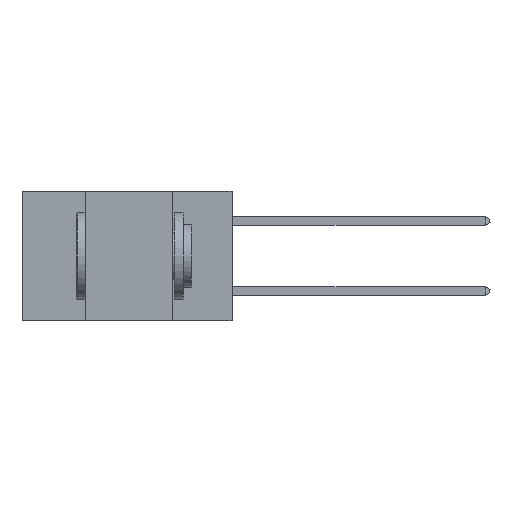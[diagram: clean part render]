
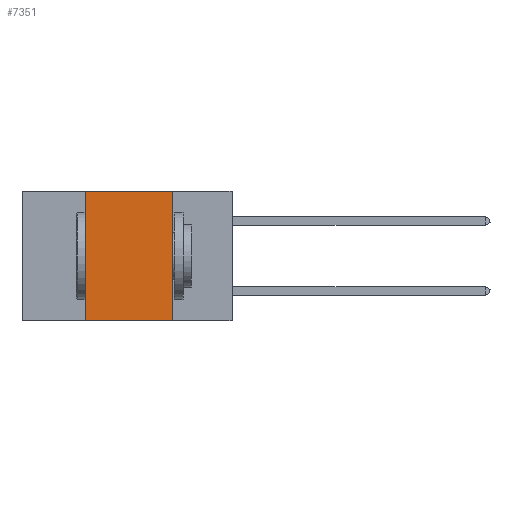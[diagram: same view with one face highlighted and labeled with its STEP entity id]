
A CAD part, left-side view. The second image highlights one B-rep face of the part: STEP entity #7351.
In plain terms, the highlighted planar face has unit normal (-1, 0, 0).
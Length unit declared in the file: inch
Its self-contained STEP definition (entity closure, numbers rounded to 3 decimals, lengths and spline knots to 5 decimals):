
#14 = CARTESIAN_POINT ( 'NONE',  ( 0., 0.6, -0.37 ) ) ;
#1125 = ORIENTED_EDGE ( 'NONE', *, *, #24568, .F. ) ;
#1738 = EDGE_CURVE ( 'NONE', #3433, #2591, #24020, .T. ) ;
#2591 = VERTEX_POINT ( 'NONE', #39258 ) ;
#2994 = VECTOR ( 'NONE', #36422, 39.37008 ) ;
#3433 = VERTEX_POINT ( 'NONE', #27072 ) ;
#7351 = ADVANCED_FACE ( 'NONE', ( #25152 ), #18467, .F. ) ;
#8470 = CARTESIAN_POINT ( 'NONE',  ( 0., 0.42, 0. ) ) ;
#8805 = VERTEX_POINT ( 'NONE', #37638 ) ;
#14696 = LINE ( 'NONE', #8470, #31044 ) ;
#15032 = ORIENTED_EDGE ( 'NONE', *, *, #27831, .F. ) ;
#15101 = DIRECTION ( 'NONE',  ( 0., 0., 1. ) ) ;
#15327 = VECTOR ( 'NONE', #28275, 39.37008 ) ;
#18467 = PLANE ( 'NONE',  #40559 ) ;
#18554 = LINE ( 'NONE', #41655, #34784 ) ;
#20506 = LINE ( 'NONE', #33242, #2994 ) ;
#20679 = ORIENTED_EDGE ( 'NONE', *, *, #38376, .F. ) ;
#21782 = DIRECTION ( 'NONE',  ( 0., 0., -1. ) ) ;
#23719 = ORIENTED_EDGE ( 'NONE', *, *, #1738, .T. ) ;
#24020 = LINE ( 'NONE', #14, #15327 ) ;
#24568 = EDGE_CURVE ( 'NONE', #8805, #2591, #18554, .T. ) ;
#25099 = EDGE_LOOP ( 'NONE', ( #1125, #20679, #15032, #23719 ) ) ;
#25152 = FACE_OUTER_BOUND ( 'NONE', #25099, .T. ) ;
#25767 = DIRECTION ( 'NONE',  ( 0., 0., -1. ) ) ;
#27072 = CARTESIAN_POINT ( 'NONE',  ( 0., 0.42, -0.37 ) ) ;
#27831 = EDGE_CURVE ( 'NONE', #3433, #28102, #14696, .T. ) ;
#28010 = CARTESIAN_POINT ( 'NONE',  ( 0., 0.6, 0. ) ) ;
#28102 = VERTEX_POINT ( 'NONE', #39347 ) ;
#28275 = DIRECTION ( 'NONE',  ( 0., -1., 0. ) ) ;
#31044 = VECTOR ( 'NONE', #15101, 39.37008 ) ;
#33242 = CARTESIAN_POINT ( 'NONE',  ( 0., 0.6, 0. ) ) ;
#34784 = VECTOR ( 'NONE', #25767, 39.37008 ) ;
#36422 = DIRECTION ( 'NONE',  ( 0., -1., 0. ) ) ;
#37638 = CARTESIAN_POINT ( 'NONE',  ( 0., 0.17, 0. ) ) ;
#38376 = EDGE_CURVE ( 'NONE', #28102, #8805, #20506, .T. ) ;
#39258 = CARTESIAN_POINT ( 'NONE',  ( 0., 0.17, -0.37 ) ) ;
#39347 = CARTESIAN_POINT ( 'NONE',  ( 0., 0.42, 0. ) ) ;
#40559 = AXIS2_PLACEMENT_3D ( 'NONE', #28010, #40958, #21782 ) ;
#40958 = DIRECTION ( 'NONE',  ( 1., 0., 0. ) ) ;
#41655 = CARTESIAN_POINT ( 'NONE',  ( 0., 0.17, 0. ) ) ;
